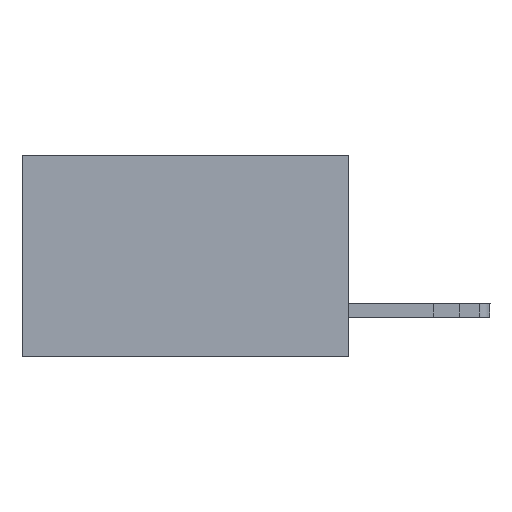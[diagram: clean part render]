
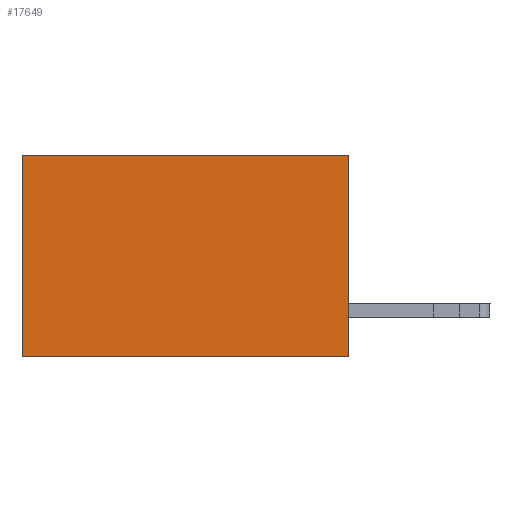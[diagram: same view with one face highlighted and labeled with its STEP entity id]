
A CAD part, left-side view. The second image highlights one B-rep face of the part: STEP entity #17649.
In plain terms, the highlighted planar face has unit normal (-1, 0, 0).
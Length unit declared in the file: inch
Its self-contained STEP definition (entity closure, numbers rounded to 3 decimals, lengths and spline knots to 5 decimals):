
#497 = VERTEX_POINT ( 'NONE', #17929 ) ;
#568 = VERTEX_POINT ( 'NONE', #7383 ) ;
#701 = DIRECTION ( 'NONE',  ( 0., 0., -1. ) ) ;
#2742 = VECTOR ( 'NONE', #701, 39.37008 ) ;
#2854 = VERTEX_POINT ( 'NONE', #14632 ) ;
#3682 = CARTESIAN_POINT ( 'NONE',  ( 0.2615, 0.6, -0.37 ) ) ;
#3715 = VECTOR ( 'NONE', #10156, 39.37008 ) ;
#3881 = LINE ( 'NONE', #4360, #20555 ) ;
#4324 = DIRECTION ( 'NONE',  ( 0., 0., -1. ) ) ;
#4360 = CARTESIAN_POINT ( 'NONE',  ( 0.2615, 0., -0.37 ) ) ;
#5744 = ORIENTED_EDGE ( 'NONE', *, *, #15193, .T. ) ;
#5883 = CARTESIAN_POINT ( 'NONE',  ( 0.2615, 0., -0.37 ) ) ;
#6436 = DIRECTION ( 'NONE',  ( 0., 0., -1. ) ) ;
#7383 = CARTESIAN_POINT ( 'NONE',  ( 0.2615, 0., 0. ) ) ;
#8651 = LINE ( 'NONE', #10444, #3715 ) ;
#9934 = EDGE_CURVE ( 'NONE', #497, #2854, #15757, .T. ) ;
#10156 = DIRECTION ( 'NONE',  ( 0., 1., 0. ) ) ;
#10444 = CARTESIAN_POINT ( 'NONE',  ( 0.2615, 0., -0.37 ) ) ;
#10522 = VECTOR ( 'NONE', #15508, 39.37008 ) ;
#10714 = ORIENTED_EDGE ( 'NONE', *, *, #11176, .F. ) ;
#11176 = EDGE_CURVE ( 'NONE', #19641, #2854, #8651, .T. ) ;
#12880 = PLANE ( 'NONE',  #14845 ) ;
#13708 = EDGE_CURVE ( 'NONE', #568, #19641, #3881, .T. ) ;
#13975 = ORIENTED_EDGE ( 'NONE', *, *, #9934, .T. ) ;
#14269 = LINE ( 'NONE', #15451, #10522 ) ;
#14489 = CARTESIAN_POINT ( 'NONE',  ( 0.2615, 0., -0.37 ) ) ;
#14632 = CARTESIAN_POINT ( 'NONE',  ( 0.2615, 0.6, -0.37 ) ) ;
#14845 = AXIS2_PLACEMENT_3D ( 'NONE', #14489, #16098, #6436 ) ;
#15193 = EDGE_CURVE ( 'NONE', #568, #497, #14269, .T. ) ;
#15451 = CARTESIAN_POINT ( 'NONE',  ( 0.2615, 0., 0. ) ) ;
#15508 = DIRECTION ( 'NONE',  ( 0., 1., 0. ) ) ;
#15665 = FACE_OUTER_BOUND ( 'NONE', #16140, .T. ) ;
#15757 = LINE ( 'NONE', #3682, #2742 ) ;
#15911 = ORIENTED_EDGE ( 'NONE', *, *, #13708, .F. ) ;
#16098 = DIRECTION ( 'NONE',  ( 1., 0., 0. ) ) ;
#16140 = EDGE_LOOP ( 'NONE', ( #13975, #10714, #15911, #5744 ) ) ;
#17649 = ADVANCED_FACE ( 'NONE', ( #15665 ), #12880, .F. ) ;
#17929 = CARTESIAN_POINT ( 'NONE',  ( 0.2615, 0.6, 0. ) ) ;
#19641 = VERTEX_POINT ( 'NONE', #5883 ) ;
#20555 = VECTOR ( 'NONE', #4324, 39.37008 ) ;
